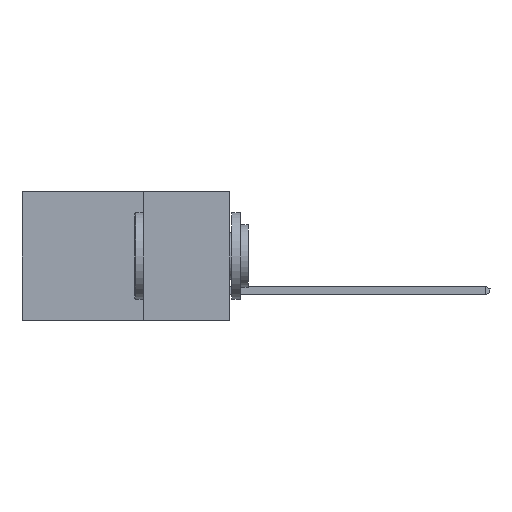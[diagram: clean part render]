
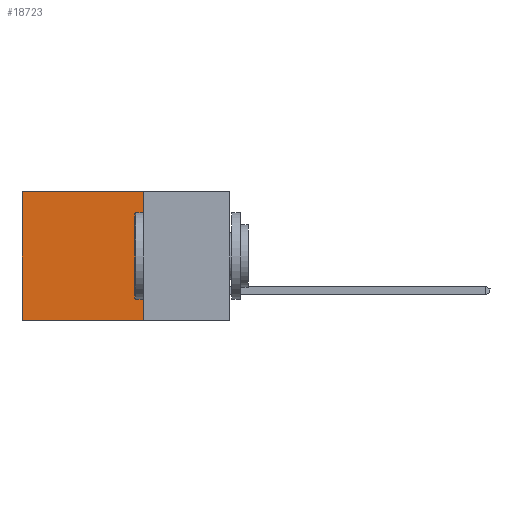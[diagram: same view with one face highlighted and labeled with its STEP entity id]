
A CAD part, left-side view. The second image highlights one B-rep face of the part: STEP entity #18723.
In plain terms, the highlighted planar face has unit normal (-1, 0, 0).
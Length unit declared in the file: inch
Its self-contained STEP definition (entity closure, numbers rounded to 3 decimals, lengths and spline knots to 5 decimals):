
#128 = AXIS2_PLACEMENT_3D ( 'NONE', #3194, #10482, #22968 ) ;
#1372 = LINE ( 'NONE', #11577, #12962 ) ;
#1548 = VERTEX_POINT ( 'NONE', #16301 ) ;
#2176 = VERTEX_POINT ( 'NONE', #16706 ) ;
#3194 = CARTESIAN_POINT ( 'NONE',  ( 0.2615, 0.25, -0.37 ) ) ;
#3859 = ORIENTED_EDGE ( 'NONE', *, *, #19916, .F. ) ;
#3912 = LINE ( 'NONE', #9107, #10821 ) ;
#3999 = CARTESIAN_POINT ( 'NONE',  ( 0.2615, 0.25, 0. ) ) ;
#4850 = EDGE_CURVE ( 'NONE', #1548, #18809, #1372, .T. ) ;
#4933 = ORIENTED_EDGE ( 'NONE', *, *, #4850, .T. ) ;
#5751 = VECTOR ( 'NONE', #13766, 39.37008 ) ;
#5848 = DIRECTION ( 'NONE',  ( 0., 1., 0. ) ) ;
#6141 = DIRECTION ( 'NONE',  ( 0., 0., -1. ) ) ;
#6658 = EDGE_CURVE ( 'NONE', #11709, #1548, #16420, .T. ) ;
#7051 = VECTOR ( 'NONE', #5848, 39.37008 ) ;
#9085 = CARTESIAN_POINT ( 'NONE',  ( 0.2615, 0.6, -0.37 ) ) ;
#9107 = CARTESIAN_POINT ( 'NONE',  ( 0.2615, 0.25, -0.37 ) ) ;
#9601 = EDGE_CURVE ( 'NONE', #2176, #18809, #3912, .T. ) ;
#10482 = DIRECTION ( 'NONE',  ( 1., 0., 0. ) ) ;
#10821 = VECTOR ( 'NONE', #14010, 39.37008 ) ;
#11577 = CARTESIAN_POINT ( 'NONE',  ( 0.2615, 0.6, -0.37 ) ) ;
#11709 = VERTEX_POINT ( 'NONE', #20943 ) ;
#12244 = ORIENTED_EDGE ( 'NONE', *, *, #9601, .F. ) ;
#12962 = VECTOR ( 'NONE', #6141, 39.37008 ) ;
#13766 = DIRECTION ( 'NONE',  ( 0., 0., -1. ) ) ;
#14010 = DIRECTION ( 'NONE',  ( 0., 1., 0. ) ) ;
#14094 = FACE_OUTER_BOUND ( 'NONE', #18777, .T. ) ;
#15043 = LINE ( 'NONE', #22279, #5751 ) ;
#15144 = ORIENTED_EDGE ( 'NONE', *, *, #6658, .T. ) ;
#16301 = CARTESIAN_POINT ( 'NONE',  ( 0.2615, 0.6, 0. ) ) ;
#16420 = LINE ( 'NONE', #3999, #7051 ) ;
#16706 = CARTESIAN_POINT ( 'NONE',  ( 0.2615, 0.25, -0.37 ) ) ;
#18723 = ADVANCED_FACE ( 'NONE', ( #14094 ), #21200, .F. ) ;
#18777 = EDGE_LOOP ( 'NONE', ( #4933, #12244, #3859, #15144 ) ) ;
#18809 = VERTEX_POINT ( 'NONE', #9085 ) ;
#19916 = EDGE_CURVE ( 'NONE', #11709, #2176, #15043, .T. ) ;
#20943 = CARTESIAN_POINT ( 'NONE',  ( 0.2615, 0.25, 0. ) ) ;
#21200 = PLANE ( 'NONE',  #128 ) ;
#22279 = CARTESIAN_POINT ( 'NONE',  ( 0.2615, 0.25, -0.37 ) ) ;
#22968 = DIRECTION ( 'NONE',  ( 0., 0., -1. ) ) ;
